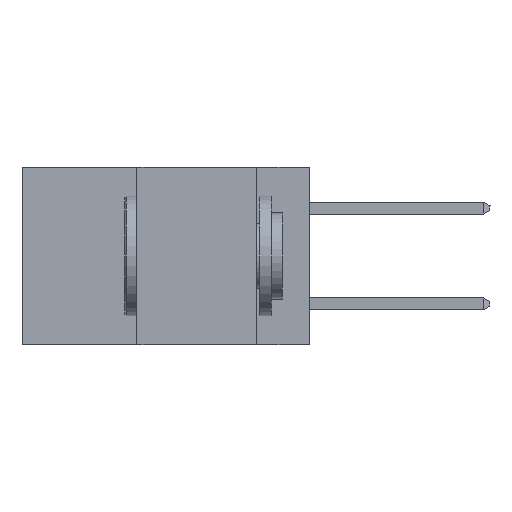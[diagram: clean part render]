
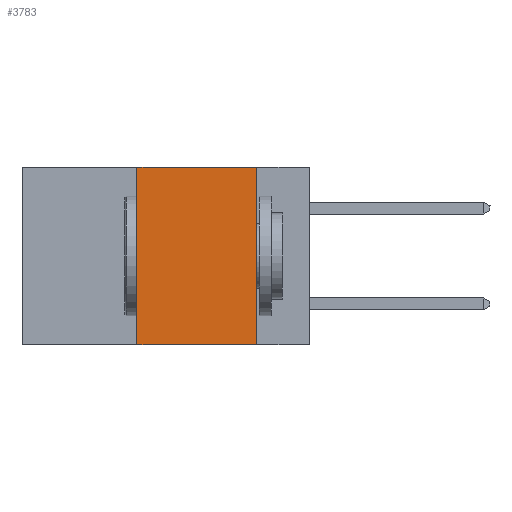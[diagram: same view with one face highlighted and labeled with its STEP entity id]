
A CAD part, left-side view. The second image highlights one B-rep face of the part: STEP entity #3783.
In plain terms, the highlighted planar face has unit normal (-1, 0, 0).
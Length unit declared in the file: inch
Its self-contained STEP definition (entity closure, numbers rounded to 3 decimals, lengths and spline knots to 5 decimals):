
#57 = VECTOR ( 'NONE', #9792, 39.37008 ) ;
#76 = DIRECTION ( 'NONE',  ( 0., 0., -1. ) ) ;
#528 = LINE ( 'NONE', #3515, #4116 ) ;
#853 = CARTESIAN_POINT ( 'NONE',  ( 0., 0.36, 0. ) ) ;
#872 = CARTESIAN_POINT ( 'NONE',  ( 0., 0.11, 0. ) ) ;
#1193 = ORIENTED_EDGE ( 'NONE', *, *, #9680, .T. ) ;
#1433 = CARTESIAN_POINT ( 'NONE',  ( 0., 0.11, -0.37 ) ) ;
#1857 = DIRECTION ( 'NONE',  ( 0., 0., 1. ) ) ;
#2067 = VERTEX_POINT ( 'NONE', #853 ) ;
#2486 = LINE ( 'NONE', #9465, #5857 ) ;
#2646 = DIRECTION ( 'NONE',  ( 0., -1., 0. ) ) ;
#2662 = ORIENTED_EDGE ( 'NONE', *, *, #7476, .F. ) ;
#3304 = VECTOR ( 'NONE', #76, 39.37008 ) ;
#3371 = FACE_OUTER_BOUND ( 'NONE', #4770, .T. ) ;
#3455 = CARTESIAN_POINT ( 'NONE',  ( 0., 0.11, 0. ) ) ;
#3515 = CARTESIAN_POINT ( 'NONE',  ( 0., 0.36, 0. ) ) ;
#3535 = ORIENTED_EDGE ( 'NONE', *, *, #10155, .F. ) ;
#3642 = VERTEX_POINT ( 'NONE', #1433 ) ;
#3783 = ADVANCED_FACE ( 'NONE', ( #3371 ), #5598, .F. ) ;
#4116 = VECTOR ( 'NONE', #1857, 39.37008 ) ;
#4770 = EDGE_LOOP ( 'NONE', ( #2662, #3535, #8823, #1193 ) ) ;
#5485 = DIRECTION ( 'NONE',  ( 1., 0., 0. ) ) ;
#5585 = LINE ( 'NONE', #872, #3304 ) ;
#5598 = PLANE ( 'NONE',  #10551 ) ;
#5857 = VECTOR ( 'NONE', #2646, 39.37008 ) ;
#6812 = VERTEX_POINT ( 'NONE', #3455 ) ;
#7176 = CARTESIAN_POINT ( 'NONE',  ( 0., 0.6, 0. ) ) ;
#7476 = EDGE_CURVE ( 'NONE', #6812, #3642, #5585, .T. ) ;
#7602 = VERTEX_POINT ( 'NONE', #9537 ) ;
#8823 = ORIENTED_EDGE ( 'NONE', *, *, #10147, .F. ) ;
#9005 = DIRECTION ( 'NONE',  ( 0., 0., -1. ) ) ;
#9465 = CARTESIAN_POINT ( 'NONE',  ( 0., 0.6, 0. ) ) ;
#9537 = CARTESIAN_POINT ( 'NONE',  ( 0., 0.36, -0.37 ) ) ;
#9680 = EDGE_CURVE ( 'NONE', #7602, #3642, #10592, .T. ) ;
#9792 = DIRECTION ( 'NONE',  ( 0., -1., 0. ) ) ;
#10147 = EDGE_CURVE ( 'NONE', #7602, #2067, #528, .T. ) ;
#10155 = EDGE_CURVE ( 'NONE', #2067, #6812, #2486, .T. ) ;
#10551 = AXIS2_PLACEMENT_3D ( 'NONE', #7176, #5485, #9005 ) ;
#10586 = CARTESIAN_POINT ( 'NONE',  ( 0., 0.6, -0.37 ) ) ;
#10592 = LINE ( 'NONE', #10586, #57 ) ;
